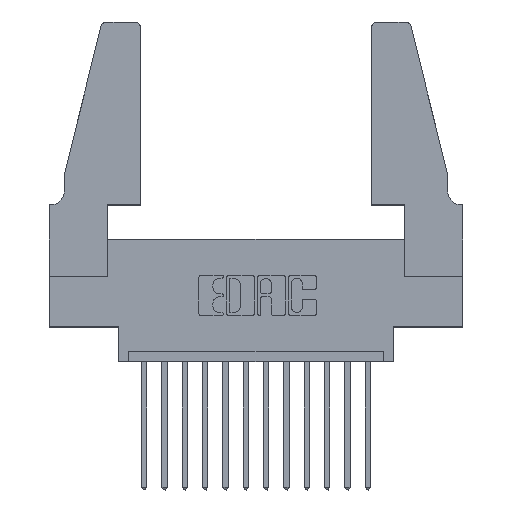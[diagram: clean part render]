
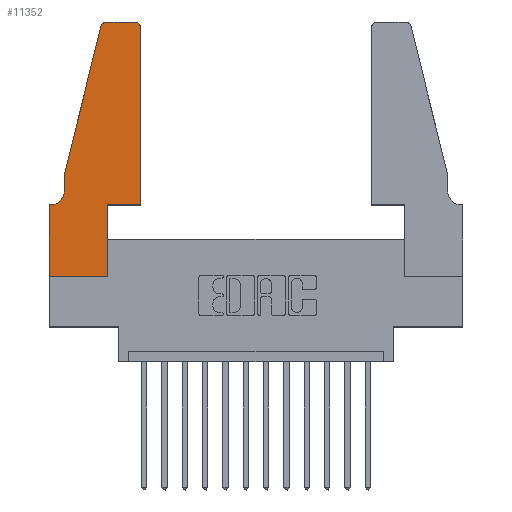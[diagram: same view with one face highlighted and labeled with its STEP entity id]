
A CAD part, top view. The second image highlights one B-rep face of the part: STEP entity #11352.
In plain terms, the highlighted planar face has unit normal (0, 0, 1).
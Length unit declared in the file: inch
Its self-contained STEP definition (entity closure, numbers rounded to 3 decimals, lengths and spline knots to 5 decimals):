
#293 = CARTESIAN_POINT ( 'NONE',  ( 0.284, 1.22, 0.37 ) ) ;
#548 = CARTESIAN_POINT ( 'NONE',  ( 0.0055, 0.42, 0.37 ) ) ;
#1018 = ORIENTED_EDGE ( 'NONE', *, *, #9961, .T. ) ;
#1265 = CARTESIAN_POINT ( 'NONE',  ( 0., 0., 0.37 ) ) ;
#1292 = LINE ( 'NONE', #11008, #3543 ) ;
#1313 = LINE ( 'NONE', #10758, #8401 ) ;
#1373 = ORIENTED_EDGE ( 'NONE', *, *, #12177, .T. ) ;
#1459 = CARTESIAN_POINT ( 'NONE',  ( 0.4505, 0.35, 0.37 ) ) ;
#1482 = DIRECTION ( 'NONE',  ( 0., 0., 1. ) ) ;
#1667 = VECTOR ( 'NONE', #5014, 39.37008 ) ;
#1745 = CARTESIAN_POINT ( 'NONE',  ( 0.284, 1.25, 0.37 ) ) ;
#1778 = CARTESIAN_POINT ( 'NONE',  ( 0.4205, 1.22, 0.37 ) ) ;
#1789 = DIRECTION ( 'NONE',  ( -1., 0., 0. ) ) ;
#2022 = DIRECTION ( 'NONE',  ( 1., 0., 0. ) ) ;
#2041 = ORIENTED_EDGE ( 'NONE', *, *, #9795, .T. ) ;
#2089 = CARTESIAN_POINT ( 'NONE',  ( 0.4505, 0.35, 0.37 ) ) ;
#2469 = CARTESIAN_POINT ( 'NONE',  ( 0., 0.35, 0.37 ) ) ;
#2502 = ORIENTED_EDGE ( 'NONE', *, *, #10729, .T. ) ;
#2524 = VERTEX_POINT ( 'NONE', #6384 ) ;
#2679 = ORIENTED_EDGE ( 'NONE', *, *, #10612, .T. ) ;
#2936 = CARTESIAN_POINT ( 'NONE',  ( 0.0755, 0.35, 0.37 ) ) ;
#3065 = VERTEX_POINT ( 'NONE', #12459 ) ;
#3391 = AXIS2_PLACEMENT_3D ( 'NONE', #548, #7780, #1789 ) ;
#3543 = VECTOR ( 'NONE', #6355, 39.37008 ) ;
#3571 = CARTESIAN_POINT ( 'NONE',  ( 0.4205, 1.25, 0.37 ) ) ;
#3725 = LINE ( 'NONE', #15189, #14319 ) ;
#3939 = VERTEX_POINT ( 'NONE', #10175 ) ;
#4422 = FACE_OUTER_BOUND ( 'NONE', #5177, .T. ) ;
#4571 = CARTESIAN_POINT ( 'NONE',  ( 0.0755, 0.5, 0.37 ) ) ;
#4627 = DIRECTION ( 'NONE',  ( 0., 1., 0. ) ) ;
#4880 = EDGE_CURVE ( 'NONE', #15284, #3065, #9179, .T. ) ;
#4900 = DIRECTION ( 'NONE',  ( 0., -1., 0. ) ) ;
#5014 = DIRECTION ( 'NONE',  ( -1., 0., 0. ) ) ;
#5177 = EDGE_LOOP ( 'NONE', ( #2041, #1373, #1018, #5904, #8056, #7560, #2679, #9336, #6230, #2502, #7985, #13883 ) ) ;
#5212 = VECTOR ( 'NONE', #7706, 39.37008 ) ;
#5292 = CIRCLE ( 'NONE', #7066, 0.03 ) ;
#5904 = ORIENTED_EDGE ( 'NONE', *, *, #15104, .T. ) ;
#6005 = EDGE_CURVE ( 'NONE', #9528, #3939, #10865, .T. ) ;
#6027 = VECTOR ( 'NONE', #13749, 39.37008 ) ;
#6230 = ORIENTED_EDGE ( 'NONE', *, *, #4880, .T. ) ;
#6271 = CARTESIAN_POINT ( 'NONE',  ( 0.2865, 0., 0.37 ) ) ;
#6355 = DIRECTION ( 'NONE',  ( -1., 0., 0. ) ) ;
#6384 = CARTESIAN_POINT ( 'NONE',  ( 0., 0.35, 0.37 ) ) ;
#6577 = DIRECTION ( 'NONE',  ( 0., 0., 1. ) ) ;
#6649 = VECTOR ( 'NONE', #8756, 39.37008 ) ;
#7066 = AXIS2_PLACEMENT_3D ( 'NONE', #1778, #6577, #14893 ) ;
#7238 = CARTESIAN_POINT ( 'NONE',  ( 0.0055, 0.35, 0.37 ) ) ;
#7360 = CARTESIAN_POINT ( 'NONE',  ( 0., 0., 0.37 ) ) ;
#7439 = EDGE_CURVE ( 'NONE', #12736, #2524, #15250, .T. ) ;
#7497 = CARTESIAN_POINT ( 'NONE',  ( 0.25487, 1.22718, 0.37 ) ) ;
#7560 = ORIENTED_EDGE ( 'NONE', *, *, #7439, .T. ) ;
#7706 = DIRECTION ( 'NONE',  ( -0.239, -0.971, 0. ) ) ;
#7780 = DIRECTION ( 'NONE',  ( 0., 0., -1. ) ) ;
#7948 = LINE ( 'NONE', #1459, #11485 ) ;
#7950 = CARTESIAN_POINT ( 'NONE',  ( 0.0755, 0.42, 0.37 ) ) ;
#7985 = ORIENTED_EDGE ( 'NONE', *, *, #6005, .T. ) ;
#8056 = ORIENTED_EDGE ( 'NONE', *, *, #9027, .T. ) ;
#8155 = LINE ( 'NONE', #7360, #6649 ) ;
#8391 = AXIS2_PLACEMENT_3D ( 'NONE', #293, #1482, #9591 ) ;
#8401 = VECTOR ( 'NONE', #4900, 39.37008 ) ;
#8520 = VERTEX_POINT ( 'NONE', #1745 ) ;
#8559 = PLANE ( 'NONE',  #13848 ) ;
#8756 = DIRECTION ( 'NONE',  ( 0., -1., 0. ) ) ;
#8904 = LINE ( 'NONE', #13729, #5212 ) ;
#9027 = EDGE_CURVE ( 'NONE', #14252, #12736, #9071, .T. ) ;
#9071 = CIRCLE ( 'NONE', #3391, 0.07 ) ;
#9099 = VERTEX_POINT ( 'NONE', #7497 ) ;
#9179 = LINE ( 'NONE', #12535, #6027 ) ;
#9336 = ORIENTED_EDGE ( 'NONE', *, *, #10073, .T. ) ;
#9409 = EDGE_CURVE ( 'NONE', #3939, #10352, #5292, .T. ) ;
#9528 = VERTEX_POINT ( 'NONE', #15052 ) ;
#9591 = DIRECTION ( 'NONE',  ( 1., 0., 0. ) ) ;
#9736 = VERTEX_POINT ( 'NONE', #1265 ) ;
#9795 = EDGE_CURVE ( 'NONE', #10352, #8520, #1292, .T. ) ;
#9961 = EDGE_CURVE ( 'NONE', #9099, #12592, #8904, .T. ) ;
#10073 = EDGE_CURVE ( 'NONE', #9736, #15284, #3725, .T. ) ;
#10175 = CARTESIAN_POINT ( 'NONE',  ( 0.4505, 1.22, 0.37 ) ) ;
#10352 = VERTEX_POINT ( 'NONE', #3571 ) ;
#10612 = EDGE_CURVE ( 'NONE', #2524, #9736, #8155, .T. ) ;
#10729 = EDGE_CURVE ( 'NONE', #3065, #9528, #7948, .T. ) ;
#10753 = DIRECTION ( 'NONE',  ( 1., 0., 0. ) ) ;
#10758 = CARTESIAN_POINT ( 'NONE',  ( 0.0755, 0.5, 0.37 ) ) ;
#10801 = DIRECTION ( 'NONE',  ( 0., 0., 1. ) ) ;
#10865 = LINE ( 'NONE', #2089, #15121 ) ;
#11008 = CARTESIAN_POINT ( 'NONE',  ( 0.2605, 1.25, 0.37 ) ) ;
#11352 = ADVANCED_FACE ( 'NONE', ( #4422 ), #8559, .T. ) ;
#11485 = VECTOR ( 'NONE', #11998, 39.37008 ) ;
#11998 = DIRECTION ( 'NONE',  ( 1., 0., 0. ) ) ;
#12177 = EDGE_CURVE ( 'NONE', #8520, #9099, #13466, .T. ) ;
#12459 = CARTESIAN_POINT ( 'NONE',  ( 0.2865, 0.35, 0.37 ) ) ;
#12535 = CARTESIAN_POINT ( 'NONE',  ( 0.2865, 0.35, 0.37 ) ) ;
#12592 = VERTEX_POINT ( 'NONE', #4571 ) ;
#12736 = VERTEX_POINT ( 'NONE', #7238 ) ;
#13466 = CIRCLE ( 'NONE', #8391, 0.03 ) ;
#13729 = CARTESIAN_POINT ( 'NONE',  ( 0.0755, 0.5, 0.37 ) ) ;
#13749 = DIRECTION ( 'NONE',  ( 0., 1., 0. ) ) ;
#13848 = AXIS2_PLACEMENT_3D ( 'NONE', #2469, #10801, #10753 ) ;
#13883 = ORIENTED_EDGE ( 'NONE', *, *, #9409, .T. ) ;
#14252 = VERTEX_POINT ( 'NONE', #7950 ) ;
#14319 = VECTOR ( 'NONE', #2022, 39.37008 ) ;
#14893 = DIRECTION ( 'NONE',  ( 1., 0., 0. ) ) ;
#15052 = CARTESIAN_POINT ( 'NONE',  ( 0.4505, 0.35, 0.37 ) ) ;
#15104 = EDGE_CURVE ( 'NONE', #12592, #14252, #1313, .T. ) ;
#15121 = VECTOR ( 'NONE', #4627, 39.37008 ) ;
#15189 = CARTESIAN_POINT ( 'NONE',  ( 0., 0., 0.37 ) ) ;
#15250 = LINE ( 'NONE', #2936, #1667 ) ;
#15284 = VERTEX_POINT ( 'NONE', #6271 ) ;
